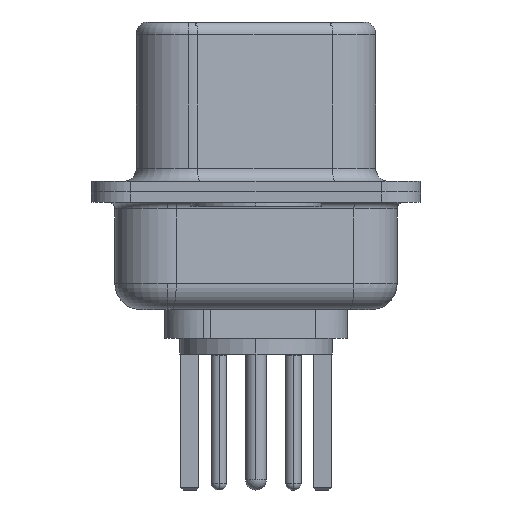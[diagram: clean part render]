
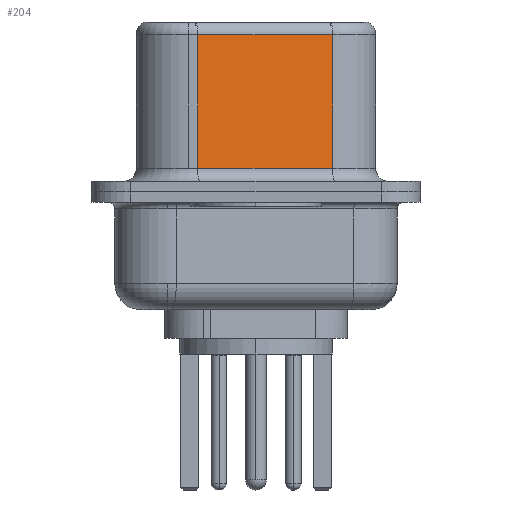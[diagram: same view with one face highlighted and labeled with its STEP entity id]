
A CAD part, left-side view. The second image highlights one B-rep face of the part: STEP entity #204.
In plain terms, the highlighted planar face has unit normal (-0.985, -0.174, 0).
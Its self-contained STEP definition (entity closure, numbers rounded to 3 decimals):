
#44 = CARTESIAN_POINT ( 'NONE',  ( 4.58, -2.927, 6.52 ) ) ;
#204 = ADVANCED_FACE ( 'NONE', ( #19896 ), #4329, .F. ) ;
#1609 = ORIENTED_EDGE ( 'NONE', *, *, #7643, .T. ) ;
#2275 = DIRECTION ( 'NONE',  ( 0., 0., -1. ) ) ;
#2540 = DIRECTION ( 'NONE',  ( 0., 0., -1. ) ) ;
#2805 = VERTEX_POINT ( 'NONE', #19477 ) ;
#3189 = CARTESIAN_POINT ( 'NONE',  ( 4.58, -2.927, 6.02 ) ) ;
#3648 = VERTEX_POINT ( 'NONE', #3189 ) ;
#4329 = PLANE ( 'NONE',  #9312 ) ;
#6141 = DIRECTION ( 'NONE',  ( -0.174, 0.985, 0. ) ) ;
#6794 = EDGE_LOOP ( 'NONE', ( #21820, #1609, #12813, #20660 ) ) ;
#7140 = LINE ( 'NONE', #19278, #20172 ) ;
#7442 = DIRECTION ( 'NONE',  ( 0.174, -0.985, 0. ) ) ;
#7493 = VERTEX_POINT ( 'NONE', #11812 ) ;
#7643 = EDGE_CURVE ( 'NONE', #3648, #17358, #18398, .T. ) ;
#8013 = DIRECTION ( 'NONE',  ( 0.985, 0.174, 0. ) ) ;
#8702 = DIRECTION ( 'NONE',  ( -0.174, 0.985, 0. ) ) ;
#9087 = EDGE_CURVE ( 'NONE', #17358, #2805, #18952, .T. ) ;
#9312 = AXIS2_PLACEMENT_3D ( 'NONE', #44, #8013, #8702 ) ;
#10810 = CARTESIAN_POINT ( 'NONE',  ( 3.67, 2.233, 6.52 ) ) ;
#11812 = CARTESIAN_POINT ( 'NONE',  ( 4.58, -2.927, 0.9 ) ) ;
#12100 = EDGE_CURVE ( 'NONE', #2805, #7493, #7140, .T. ) ;
#12813 = ORIENTED_EDGE ( 'NONE', *, *, #9087, .T. ) ;
#14381 = VECTOR ( 'NONE', #2275, 1000. ) ;
#14480 = CARTESIAN_POINT ( 'NONE',  ( 4.58, -2.927, 6.52 ) ) ;
#15512 = CARTESIAN_POINT ( 'NONE',  ( 3.67, 2.233, 6.02 ) ) ;
#16719 = EDGE_CURVE ( 'NONE', #3648, #7493, #17214, .T. ) ;
#17214 = LINE ( 'NONE', #14480, #21190 ) ;
#17358 = VERTEX_POINT ( 'NONE', #15512 ) ;
#17859 = VECTOR ( 'NONE', #6141, 1000. ) ;
#18398 = LINE ( 'NONE', #19936, #17859 ) ;
#18952 = LINE ( 'NONE', #10810, #14381 ) ;
#19278 = CARTESIAN_POINT ( 'NONE',  ( 4.58, -2.927, 0.9 ) ) ;
#19477 = CARTESIAN_POINT ( 'NONE',  ( 3.67, 2.233, 0.9 ) ) ;
#19896 = FACE_OUTER_BOUND ( 'NONE', #6794, .T. ) ;
#19936 = CARTESIAN_POINT ( 'NONE',  ( 4.58, -2.927, 6.02 ) ) ;
#20172 = VECTOR ( 'NONE', #7442, 1000. ) ;
#20660 = ORIENTED_EDGE ( 'NONE', *, *, #12100, .T. ) ;
#21190 = VECTOR ( 'NONE', #2540, 1000. ) ;
#21820 = ORIENTED_EDGE ( 'NONE', *, *, #16719, .F. ) ;
